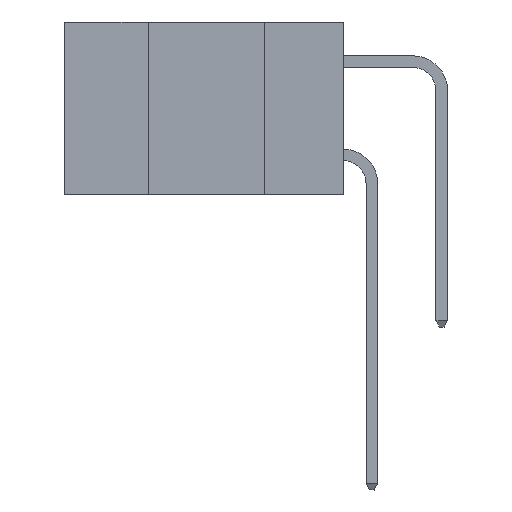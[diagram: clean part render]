
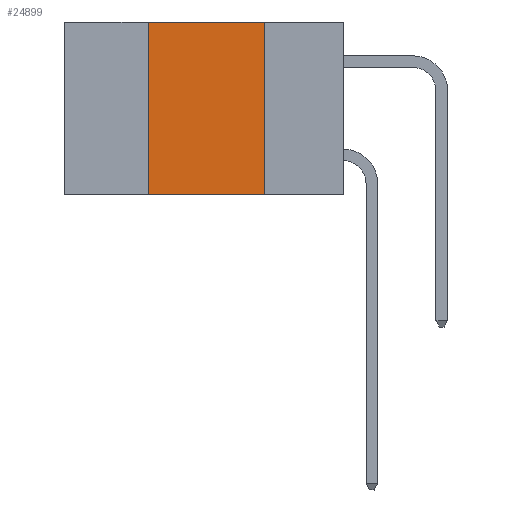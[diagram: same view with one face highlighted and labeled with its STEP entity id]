
A CAD part, left-side view. The second image highlights one B-rep face of the part: STEP entity #24899.
In plain terms, the highlighted planar face has unit normal (-1, 0, 0).
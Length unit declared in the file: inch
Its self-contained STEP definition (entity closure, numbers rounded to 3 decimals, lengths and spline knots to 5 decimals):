
#262 = LINE ( 'NONE', #23688, #5483 ) ;
#1015 = ORIENTED_EDGE ( 'NONE', *, *, #9855, .T. ) ;
#1337 = VECTOR ( 'NONE', #11767, 39.37008 ) ;
#1495 = EDGE_CURVE ( 'NONE', #14138, #8181, #24965, .T. ) ;
#2855 = ORIENTED_EDGE ( 'NONE', *, *, #20923, .F. ) ;
#4293 = CARTESIAN_POINT ( 'NONE',  ( 0., 0.17, 0. ) ) ;
#5483 = VECTOR ( 'NONE', #19977, 39.37008 ) ;
#8181 = VERTEX_POINT ( 'NONE', #9983 ) ;
#8370 = DIRECTION ( 'NONE',  ( 0., 0., 1. ) ) ;
#9258 = LINE ( 'NONE', #16214, #24927 ) ;
#9855 = EDGE_CURVE ( 'NONE', #10480, #8181, #262, .T. ) ;
#9983 = CARTESIAN_POINT ( 'NONE',  ( 0., 0.17, -0.37 ) ) ;
#10058 = ORIENTED_EDGE ( 'NONE', *, *, #1495, .F. ) ;
#10321 = CARTESIAN_POINT ( 'NONE',  ( 0., 0.42, 0. ) ) ;
#10480 = VERTEX_POINT ( 'NONE', #23580 ) ;
#11048 = CARTESIAN_POINT ( 'NONE',  ( 0., 0.6, 0. ) ) ;
#11073 = EDGE_LOOP ( 'NONE', ( #10058, #19204, #2855, #1015 ) ) ;
#11767 = DIRECTION ( 'NONE',  ( 0., 0., -1. ) ) ;
#13203 = VECTOR ( 'NONE', #8370, 39.37008 ) ;
#14138 = VERTEX_POINT ( 'NONE', #4293 ) ;
#14141 = FACE_OUTER_BOUND ( 'NONE', #11073, .T. ) ;
#14207 = VERTEX_POINT ( 'NONE', #10321 ) ;
#14495 = DIRECTION ( 'NONE',  ( 0., -1., 0. ) ) ;
#15946 = LINE ( 'NONE', #18113, #13203 ) ;
#16214 = CARTESIAN_POINT ( 'NONE',  ( 0., 0.6, 0. ) ) ;
#17557 = CARTESIAN_POINT ( 'NONE',  ( 0., 0.17, 0. ) ) ;
#18113 = CARTESIAN_POINT ( 'NONE',  ( 0., 0.42, 0. ) ) ;
#19204 = ORIENTED_EDGE ( 'NONE', *, *, #19976, .F. ) ;
#19976 = EDGE_CURVE ( 'NONE', #14207, #14138, #9258, .T. ) ;
#19977 = DIRECTION ( 'NONE',  ( 0., -1., 0. ) ) ;
#20529 = DIRECTION ( 'NONE',  ( 1., 0., 0. ) ) ;
#20923 = EDGE_CURVE ( 'NONE', #10480, #14207, #15946, .T. ) ;
#22301 = AXIS2_PLACEMENT_3D ( 'NONE', #11048, #20529, #24757 ) ;
#23580 = CARTESIAN_POINT ( 'NONE',  ( 0., 0.42, -0.37 ) ) ;
#23688 = CARTESIAN_POINT ( 'NONE',  ( 0., 0.6, -0.37 ) ) ;
#24757 = DIRECTION ( 'NONE',  ( 0., 0., -1. ) ) ;
#24854 = PLANE ( 'NONE',  #22301 ) ;
#24899 = ADVANCED_FACE ( 'NONE', ( #14141 ), #24854, .F. ) ;
#24927 = VECTOR ( 'NONE', #14495, 39.37008 ) ;
#24965 = LINE ( 'NONE', #17557, #1337 ) ;
